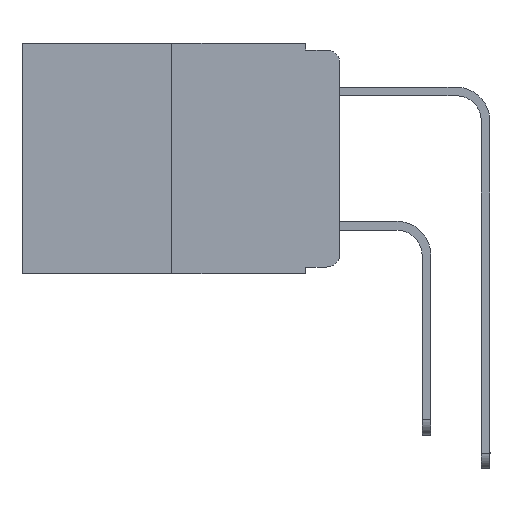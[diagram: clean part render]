
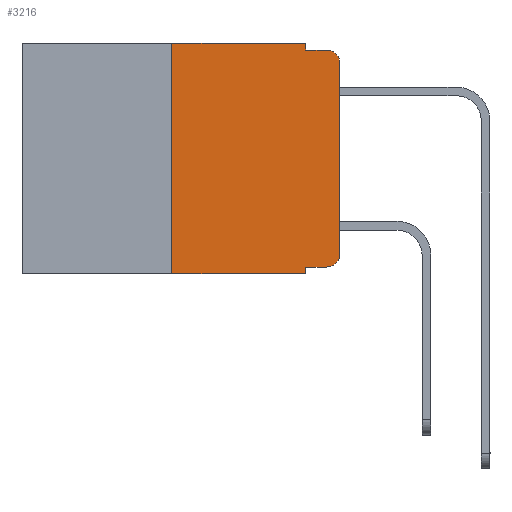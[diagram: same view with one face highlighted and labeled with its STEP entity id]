
A CAD part, left-side view. The second image highlights one B-rep face of the part: STEP entity #3216.
In plain terms, the highlighted planar face has unit normal (-1, 0, 0).
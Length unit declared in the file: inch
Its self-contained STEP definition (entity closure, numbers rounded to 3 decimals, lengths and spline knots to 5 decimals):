
#115 = DIRECTION ( 'NONE',  ( 0., 0., -1. ) ) ;
#145 = VERTEX_POINT ( 'NONE', #6567 ) ;
#212 = CIRCLE ( 'NONE', #13137, 0.02 ) ;
#294 = EDGE_CURVE ( 'NONE', #8805, #10127, #3382, .T. ) ;
#400 = DIRECTION ( 'NONE',  ( 0., 0., -1. ) ) ;
#666 = DIRECTION ( 'NONE',  ( 0., -1., 0. ) ) ;
#946 = ORIENTED_EDGE ( 'NONE', *, *, #2915, .F. ) ;
#1159 = VECTOR ( 'NONE', #115, 39.37008 ) ;
#1263 = CARTESIAN_POINT ( 'NONE',  ( 0., 0.02, -0.03 ) ) ;
#1286 = VECTOR ( 'NONE', #6414, 39.37008 ) ;
#1409 = ORIENTED_EDGE ( 'NONE', *, *, #9854, .F. ) ;
#1462 = LINE ( 'NONE', #12519, #4007 ) ;
#2027 = EDGE_CURVE ( 'NONE', #7018, #5141, #8538, .T. ) ;
#2186 = VERTEX_POINT ( 'NONE', #6594 ) ;
#2286 = DIRECTION ( 'NONE',  ( 0., 0., -1. ) ) ;
#2546 = VECTOR ( 'NONE', #11094, 39.37008 ) ;
#2606 = VECTOR ( 'NONE', #6243, 39.37008 ) ;
#2915 = EDGE_CURVE ( 'NONE', #11255, #2186, #7359, .T. ) ;
#2938 = ORIENTED_EDGE ( 'NONE', *, *, #5032, .F. ) ;
#2969 = LINE ( 'NONE', #11777, #8261 ) ;
#3216 = ADVANCED_FACE ( 'NONE', ( #8146 ), #13717, .F. ) ;
#3382 = LINE ( 'NONE', #12175, #2546 ) ;
#3482 = AXIS2_PLACEMENT_3D ( 'NONE', #11659, #11596, #5107 ) ;
#3859 = AXIS2_PLACEMENT_3D ( 'NONE', #6846, #8204, #400 ) ;
#4007 = VECTOR ( 'NONE', #8180, 39.37008 ) ;
#4145 = CARTESIAN_POINT ( 'NONE',  ( 0., 0.473, -0.343 ) ) ;
#4226 = ORIENTED_EDGE ( 'NONE', *, *, #7242, .T. ) ;
#4684 = DIRECTION ( 'NONE',  ( -1., 0., 0. ) ) ;
#4768 = VERTEX_POINT ( 'NONE', #5385 ) ;
#4831 = ORIENTED_EDGE ( 'NONE', *, *, #2027, .T. ) ;
#5032 = EDGE_CURVE ( 'NONE', #10396, #13932, #11713, .T. ) ;
#5107 = DIRECTION ( 'NONE',  ( 0., 0., -1. ) ) ;
#5141 = VERTEX_POINT ( 'NONE', #7262 ) ;
#5385 = CARTESIAN_POINT ( 'NONE',  ( 0., 0., -0.03 ) ) ;
#5412 = EDGE_LOOP ( 'NONE', ( #11909, #10061, #946, #1409, #2938, #9956, #4831, #7176, #11529, #4226 ) ) ;
#5673 = CARTESIAN_POINT ( 'NONE',  ( 0., 0.25, 0. ) ) ;
#6085 = CARTESIAN_POINT ( 'NONE',  ( 0., 0.02, -0.333 ) ) ;
#6243 = DIRECTION ( 'NONE',  ( 0., -1., 0. ) ) ;
#6414 = DIRECTION ( 'NONE',  ( 0., -1., 0. ) ) ;
#6567 = CARTESIAN_POINT ( 'NONE',  ( 0., 0., -0.313 ) ) ;
#6594 = CARTESIAN_POINT ( 'NONE',  ( 0., 0.02, -0.01 ) ) ;
#6632 = LINE ( 'NONE', #11009, #1159 ) ;
#6787 = LINE ( 'NONE', #7866, #8326 ) ;
#6846 = CARTESIAN_POINT ( 'NONE',  ( 0., 0.473, 0. ) ) ;
#7018 = VERTEX_POINT ( 'NONE', #9149 ) ;
#7073 = EDGE_CURVE ( 'NONE', #8805, #5141, #6632, .T. ) ;
#7176 = ORIENTED_EDGE ( 'NONE', *, *, #7073, .F. ) ;
#7242 = EDGE_CURVE ( 'NONE', #10127, #145, #12928, .T. ) ;
#7262 = CARTESIAN_POINT ( 'NONE',  ( 0., 0.051, -0.343 ) ) ;
#7359 = LINE ( 'NONE', #12777, #1286 ) ;
#7866 = CARTESIAN_POINT ( 'NONE',  ( 0., 0.25, 0. ) ) ;
#7934 = CARTESIAN_POINT ( 'NONE',  ( 0., 0.051, 0. ) ) ;
#8146 = FACE_OUTER_BOUND ( 'NONE', #5412, .T. ) ;
#8180 = DIRECTION ( 'NONE',  ( 0., 0., 1. ) ) ;
#8204 = DIRECTION ( 'NONE',  ( 1., 0., 0. ) ) ;
#8261 = VECTOR ( 'NONE', #10683, 39.37008 ) ;
#8326 = VECTOR ( 'NONE', #12257, 39.37008 ) ;
#8538 = LINE ( 'NONE', #4145, #2606 ) ;
#8805 = VERTEX_POINT ( 'NONE', #8996 ) ;
#8996 = CARTESIAN_POINT ( 'NONE',  ( 0., 0.051, -0.333 ) ) ;
#9149 = CARTESIAN_POINT ( 'NONE',  ( 0., 0.25, -0.343 ) ) ;
#9323 = EDGE_CURVE ( 'NONE', #145, #4768, #1462, .T. ) ;
#9854 = EDGE_CURVE ( 'NONE', #13932, #11255, #2969, .T. ) ;
#9902 = CARTESIAN_POINT ( 'NONE',  ( 0., 0.051, -0.01 ) ) ;
#9956 = ORIENTED_EDGE ( 'NONE', *, *, #14048, .F. ) ;
#10061 = ORIENTED_EDGE ( 'NONE', *, *, #13319, .T. ) ;
#10127 = VERTEX_POINT ( 'NONE', #6085 ) ;
#10396 = VERTEX_POINT ( 'NONE', #5673 ) ;
#10683 = DIRECTION ( 'NONE',  ( 0., 0., -1. ) ) ;
#11009 = CARTESIAN_POINT ( 'NONE',  ( 0., 0.051, 0. ) ) ;
#11094 = DIRECTION ( 'NONE',  ( 0., -1., 0. ) ) ;
#11255 = VERTEX_POINT ( 'NONE', #9902 ) ;
#11529 = ORIENTED_EDGE ( 'NONE', *, *, #294, .T. ) ;
#11596 = DIRECTION ( 'NONE',  ( -1., 0., 0. ) ) ;
#11659 = CARTESIAN_POINT ( 'NONE',  ( 0., 0.02, -0.313 ) ) ;
#11713 = LINE ( 'NONE', #13843, #13567 ) ;
#11777 = CARTESIAN_POINT ( 'NONE',  ( 0., 0.051, 0. ) ) ;
#11909 = ORIENTED_EDGE ( 'NONE', *, *, #9323, .T. ) ;
#12175 = CARTESIAN_POINT ( 'NONE',  ( 0., 0.051, -0.333 ) ) ;
#12257 = DIRECTION ( 'NONE',  ( 0., 0., 1. ) ) ;
#12519 = CARTESIAN_POINT ( 'NONE',  ( 0., 0., 0. ) ) ;
#12777 = CARTESIAN_POINT ( 'NONE',  ( 0., 0.051, -0.01 ) ) ;
#12928 = CIRCLE ( 'NONE', #3482, 0.02 ) ;
#13137 = AXIS2_PLACEMENT_3D ( 'NONE', #1263, #4684, #2286 ) ;
#13319 = EDGE_CURVE ( 'NONE', #4768, #2186, #212, .T. ) ;
#13567 = VECTOR ( 'NONE', #666, 39.37008 ) ;
#13717 = PLANE ( 'NONE',  #3859 ) ;
#13843 = CARTESIAN_POINT ( 'NONE',  ( 0., 0.473, 0. ) ) ;
#13932 = VERTEX_POINT ( 'NONE', #7934 ) ;
#14048 = EDGE_CURVE ( 'NONE', #7018, #10396, #6787, .T. ) ;
